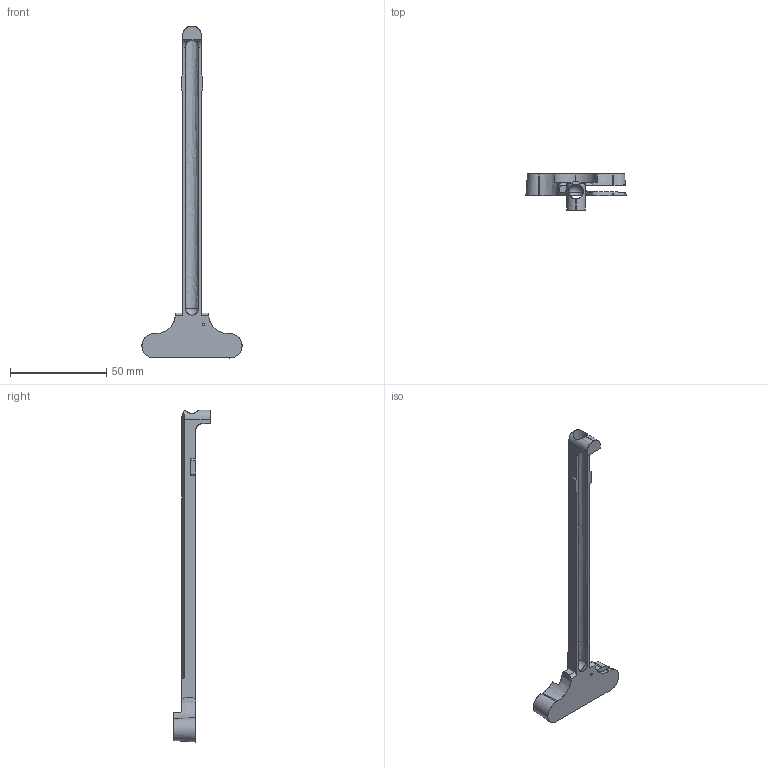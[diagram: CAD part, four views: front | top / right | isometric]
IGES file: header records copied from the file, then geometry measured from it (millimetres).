
Start section: SolidWorks IGES file using analytic representation for surfaces
Global section: file name: AR charging handle.IGS; native system: SolidWorks 2008; preprocessor: SolidWorks 2008; author: owner; date: 110706.151311; units: inch
Bounding box: 52.07 x 19.05 x 172.59 mm (x, y, z)
Surface area: 10310.5 mm2 (no closed solid volume)
Topology: 0 solids, 0 shells, 423 faces, 5321 edges, 5321 vertices
Faces by surface type: bspline 400, revolution 23
